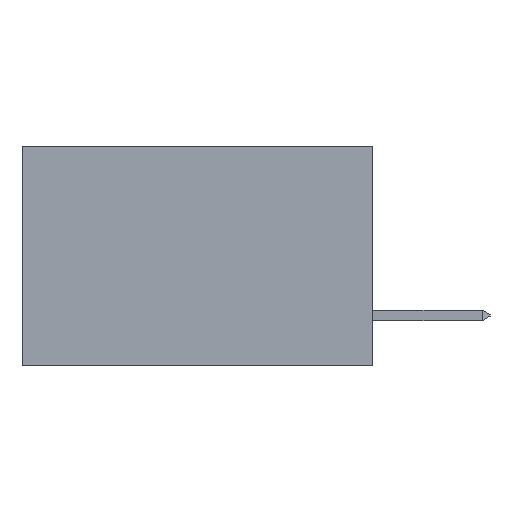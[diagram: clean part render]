
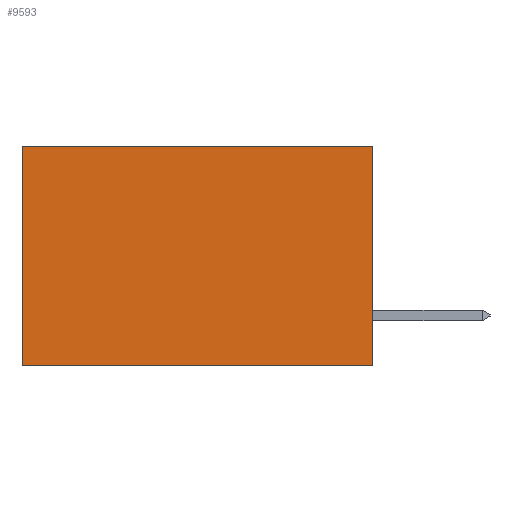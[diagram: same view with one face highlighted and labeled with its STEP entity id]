
A CAD part, left-side view. The second image highlights one B-rep face of the part: STEP entity #9593.
In plain terms, the highlighted planar face has unit normal (-1, 0, 0).
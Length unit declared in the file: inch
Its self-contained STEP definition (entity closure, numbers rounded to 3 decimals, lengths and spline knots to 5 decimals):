
#468 = EDGE_LOOP ( 'NONE', ( #9301, #10018, #3595, #3768 ) ) ;
#891 = PLANE ( 'NONE',  #12691 ) ;
#978 = VERTEX_POINT ( 'NONE', #4487 ) ;
#1992 = CARTESIAN_POINT ( 'NONE',  ( 0.277, 0., -0.37 ) ) ;
#2122 = FACE_OUTER_BOUND ( 'NONE', #468, .T. ) ;
#2211 = LINE ( 'NONE', #8654, #2559 ) ;
#2559 = VECTOR ( 'NONE', #8895, 39.37008 ) ;
#2818 = EDGE_CURVE ( 'NONE', #978, #8864, #11367, .T. ) ;
#3050 = DIRECTION ( 'NONE',  ( 0., 0., -1. ) ) ;
#3595 = ORIENTED_EDGE ( 'NONE', *, *, #3668, .F. ) ;
#3668 = EDGE_CURVE ( 'NONE', #6909, #6907, #11964, .T. ) ;
#3768 = ORIENTED_EDGE ( 'NONE', *, *, #12777, .T. ) ;
#4487 = CARTESIAN_POINT ( 'NONE',  ( 0.277, 0.59, 0. ) ) ;
#5108 = CARTESIAN_POINT ( 'NONE',  ( 0.277, 0., -0.37 ) ) ;
#5723 = CARTESIAN_POINT ( 'NONE',  ( 0.277, 0., 0. ) ) ;
#5940 = CARTESIAN_POINT ( 'NONE',  ( 0.277, 0.59, -0.37 ) ) ;
#6044 = CARTESIAN_POINT ( 'NONE',  ( 0.277, 0.59, -0.37 ) ) ;
#6414 = EDGE_CURVE ( 'NONE', #6907, #8864, #2211, .T. ) ;
#6745 = CARTESIAN_POINT ( 'NONE',  ( 0.277, 0., 0. ) ) ;
#6907 = VERTEX_POINT ( 'NONE', #5108 ) ;
#6909 = VERTEX_POINT ( 'NONE', #5723 ) ;
#8654 = CARTESIAN_POINT ( 'NONE',  ( 0.277, 0., -0.37 ) ) ;
#8676 = VECTOR ( 'NONE', #11513, 39.37008 ) ;
#8864 = VERTEX_POINT ( 'NONE', #6044 ) ;
#8895 = DIRECTION ( 'NONE',  ( 0., 1., 0. ) ) ;
#9203 = DIRECTION ( 'NONE',  ( 1., 0., 0. ) ) ;
#9301 = ORIENTED_EDGE ( 'NONE', *, *, #2818, .T. ) ;
#9593 = ADVANCED_FACE ( 'NONE', ( #2122 ), #891, .F. ) ;
#9600 = VECTOR ( 'NONE', #11026, 39.37008 ) ;
#10018 = ORIENTED_EDGE ( 'NONE', *, *, #6414, .F. ) ;
#10085 = VECTOR ( 'NONE', #11756, 39.37008 ) ;
#10860 = CARTESIAN_POINT ( 'NONE',  ( 0.277, 0., -0.37 ) ) ;
#11026 = DIRECTION ( 'NONE',  ( 0., 0., -1. ) ) ;
#11367 = LINE ( 'NONE', #5940, #8676 ) ;
#11513 = DIRECTION ( 'NONE',  ( 0., 0., -1. ) ) ;
#11756 = DIRECTION ( 'NONE',  ( 0., 1., 0. ) ) ;
#11964 = LINE ( 'NONE', #10860, #9600 ) ;
#12691 = AXIS2_PLACEMENT_3D ( 'NONE', #1992, #9203, #3050 ) ;
#12777 = EDGE_CURVE ( 'NONE', #6909, #978, #13060, .T. ) ;
#13060 = LINE ( 'NONE', #6745, #10085 ) ;
